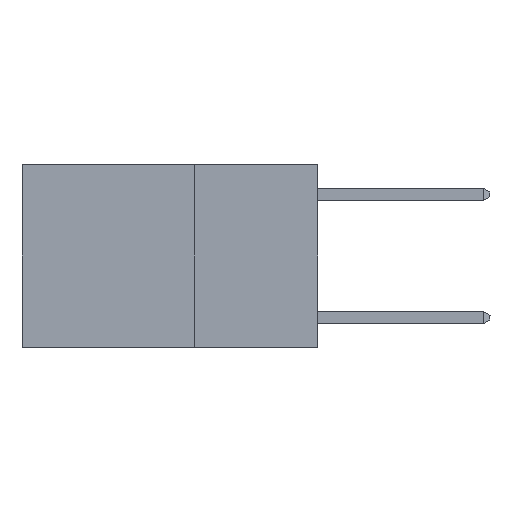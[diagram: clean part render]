
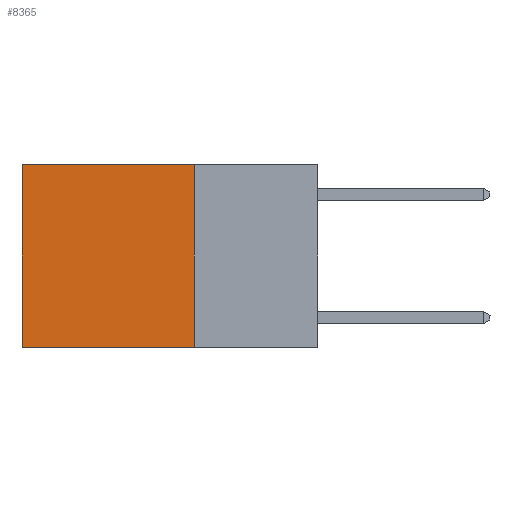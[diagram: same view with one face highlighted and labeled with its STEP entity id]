
A CAD part, left-side view. The second image highlights one B-rep face of the part: STEP entity #8365.
In plain terms, the highlighted planar face has unit normal (-1, 0, 0).
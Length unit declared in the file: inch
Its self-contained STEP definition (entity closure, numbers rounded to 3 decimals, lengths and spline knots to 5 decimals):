
#35 = DIRECTION ( 'NONE',  ( 0., 1., 0. ) ) ;
#250 = EDGE_LOOP ( 'NONE', ( #11408, #15784, #9503, #8236 ) ) ;
#840 = LINE ( 'NONE', #8207, #4060 ) ;
#1078 = CARTESIAN_POINT ( 'NONE',  ( 0.2625, 0.25, 0. ) ) ;
#1190 = VERTEX_POINT ( 'NONE', #2785 ) ;
#1417 = VERTEX_POINT ( 'NONE', #17675 ) ;
#1799 = VECTOR ( 'NONE', #35, 39.37008 ) ;
#2556 = CARTESIAN_POINT ( 'NONE',  ( 0.2625, 0.25, 0. ) ) ;
#2769 = CARTESIAN_POINT ( 'NONE',  ( 0.2625, 0.25, -0.37 ) ) ;
#2785 = CARTESIAN_POINT ( 'NONE',  ( 0.2625, 0.25, -0.37 ) ) ;
#3809 = DIRECTION ( 'NONE',  ( 0., 0., -1. ) ) ;
#4060 = VECTOR ( 'NONE', #3809, 39.37008 ) ;
#4167 = EDGE_CURVE ( 'NONE', #1417, #10535, #840, .T. ) ;
#5228 = VECTOR ( 'NONE', #14553, 39.37008 ) ;
#5505 = LINE ( 'NONE', #2556, #1799 ) ;
#6375 = VERTEX_POINT ( 'NONE', #1078 ) ;
#6451 = EDGE_CURVE ( 'NONE', #6375, #1417, #5505, .T. ) ;
#7657 = CARTESIAN_POINT ( 'NONE',  ( 0.2625, 0.25, 0. ) ) ;
#8207 = CARTESIAN_POINT ( 'NONE',  ( 0.2625, 0.6, 0. ) ) ;
#8236 = ORIENTED_EDGE ( 'NONE', *, *, #6451, .T. ) ;
#8340 = VECTOR ( 'NONE', #15328, 39.37008 ) ;
#8365 = ADVANCED_FACE ( 'NONE', ( #12900 ), #17210, .F. ) ;
#9503 = ORIENTED_EDGE ( 'NONE', *, *, #17986, .F. ) ;
#9952 = LINE ( 'NONE', #2769, #8340 ) ;
#10101 = CARTESIAN_POINT ( 'NONE',  ( 0.2625, 0.6, -0.37 ) ) ;
#10535 = VERTEX_POINT ( 'NONE', #10101 ) ;
#11408 = ORIENTED_EDGE ( 'NONE', *, *, #4167, .T. ) ;
#11805 = DIRECTION ( 'NONE',  ( 1., 0., 0. ) ) ;
#11870 = EDGE_CURVE ( 'NONE', #1190, #10535, #9952, .T. ) ;
#11964 = DIRECTION ( 'NONE',  ( 0., 0., -1. ) ) ;
#12900 = FACE_OUTER_BOUND ( 'NONE', #250, .T. ) ;
#13044 = CARTESIAN_POINT ( 'NONE',  ( 0.2625, 0.25, 0. ) ) ;
#14077 = AXIS2_PLACEMENT_3D ( 'NONE', #7657, #11805, #11964 ) ;
#14553 = DIRECTION ( 'NONE',  ( 0., 0., -1. ) ) ;
#15328 = DIRECTION ( 'NONE',  ( 0., 1., 0. ) ) ;
#15784 = ORIENTED_EDGE ( 'NONE', *, *, #11870, .F. ) ;
#17210 = PLANE ( 'NONE',  #14077 ) ;
#17346 = LINE ( 'NONE', #13044, #5228 ) ;
#17675 = CARTESIAN_POINT ( 'NONE',  ( 0.2625, 0.6, 0. ) ) ;
#17986 = EDGE_CURVE ( 'NONE', #6375, #1190, #17346, .T. ) ;
